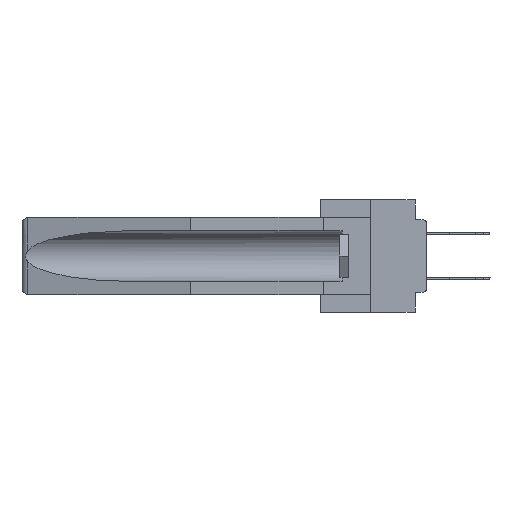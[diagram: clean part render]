
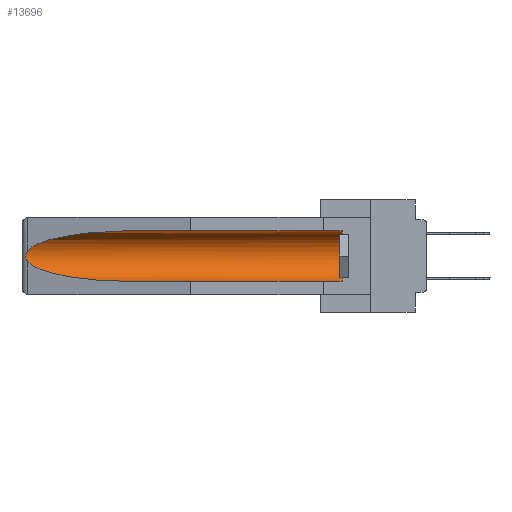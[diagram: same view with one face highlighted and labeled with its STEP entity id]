
A CAD part, left-side view. The second image highlights one B-rep face of the part: STEP entity #13696.
In plain terms, the highlighted cylindrical face has radius 2.857 mm (diameter 5.715 mm), a partial arc.
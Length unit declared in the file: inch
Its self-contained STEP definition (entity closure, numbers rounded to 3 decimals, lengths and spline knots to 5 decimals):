
#3697 = CARTESIAN_POINT ( 'NONE',  ( 0.25451, 1.48313, -0.09465 ) ) ;
#4041 = CARTESIAN_POINT ( 'NONE',  ( 0.26537, 1.52718, -0.14972 ) ) ;
#4140 = CARTESIAN_POINT ( 'NONE',  ( 0.26537, 1.52718, -0.19328 ) ) ;
#4687 = DIRECTION ( 'NONE',  ( 0., 1., 0. ) ) ;
#4761 = EDGE_CURVE ( 'NONE', #7345, #20458, #6407, .T. ) ;
#4946 = B_SPLINE_CURVE_WITH_KNOTS ( 'NONE', 3,
 ( #4041, #6804, #26663, #19474, #11679, #11792, #11461, #6586, #21898, #4140 ),
 .UNSPECIFIED., .F., .F.,
 ( 4, 2, 2, 2, 4 ),
 ( 0., 0.00029, 0.00058, 0.00087, 0.00117 ),
 .UNSPECIFIED. ) ;
#5360 = CARTESIAN_POINT ( 'NONE',  ( 0.155, -0.30754, -0.059 ) ) ;
#5689 = CARTESIAN_POINT ( 'NONE',  ( 0.26537, 1.52718, -0.19328 ) ) ;
#6020 = VERTEX_POINT ( 'NONE', #6176 ) ;
#6176 = CARTESIAN_POINT ( 'NONE',  ( 0.155, 0.126, -0.059 ) ) ;
#6407 = LINE ( 'NONE', #17045, #32652 ) ;
#6586 = CARTESIAN_POINT ( 'NONE',  ( 0.26655, 1.53094, -0.18657 ) ) ;
#6804 = CARTESIAN_POINT ( 'NONE',  ( 0.26597, 1.52961, -0.15275 ) ) ;
#7345 = VERTEX_POINT ( 'NONE', #15353 ) ;
#8483 = ORIENTED_EDGE ( 'NONE', *, *, #4761, .F. ) ;
#9183 = EDGE_CURVE ( 'NONE', #24063, #11106, #10831, .T. ) ;
#9950 = LINE ( 'NONE', #5360, #30214 ) ;
#10102 = EDGE_CURVE ( 'NONE', #7345, #6020, #14023, .T. ) ;
#10831 =( BOUNDED_CURVE ( )  B_SPLINE_CURVE ( 3, ( #16141, #11220, #3697, #11896 ),
 .UNSPECIFIED., .F., .F. ) 
 B_SPLINE_CURVE_WITH_KNOTS ( ( 4, 4 ),
 ( 4.71239, 6.08839 ),
 .UNSPECIFIED. ) 
 CURVE ( )  GEOMETRIC_REPRESENTATION_ITEM ( )  RATIONAL_B_SPLINE_CURVE ( ( 1., 0.848, 0.848, 1. ) ) 
 REPRESENTATION_ITEM ( '' )  );
#11016 = VERTEX_POINT ( 'NONE', #11349 ) ;
#11106 = VERTEX_POINT ( 'NONE', #11783 ) ;
#11220 = CARTESIAN_POINT ( 'NONE',  ( 0.21114, 1.30732, -0.059 ) ) ;
#11349 = CARTESIAN_POINT ( 'NONE',  ( 0.26537, 1.52718, -0.19328 ) ) ;
#11461 = CARTESIAN_POINT ( 'NONE',  ( 0.2673, 1.53269, -0.17917 ) ) ;
#11679 = CARTESIAN_POINT ( 'NONE',  ( 0.2675, 1.53308, -0.16763 ) ) ;
#11783 = CARTESIAN_POINT ( 'NONE',  ( 0.26537, 1.52718, -0.14972 ) ) ;
#11792 = CARTESIAN_POINT ( 'NONE',  ( 0.2675, 1.53308, -0.17534 ) ) ;
#11862 =( BOUNDED_CURVE ( )  B_SPLINE_CURVE ( 3, ( #5689, #23330, #28412, #21090 ),
 .UNSPECIFIED., .F., .F. ) 
 B_SPLINE_CURVE_WITH_KNOTS ( ( 4, 4 ),
 ( 0.1948, 1.5708 ),
 .UNSPECIFIED. ) 
 CURVE ( )  GEOMETRIC_REPRESENTATION_ITEM ( )  RATIONAL_B_SPLINE_CURVE ( ( 1., 0.848, 0.848, 1. ) ) 
 REPRESENTATION_ITEM ( '' )  );
#11896 = CARTESIAN_POINT ( 'NONE',  ( 0.26537, 1.52718, -0.14972 ) ) ;
#12158 = DIRECTION ( 'NONE',  ( 0., 1., 0. ) ) ;
#12189 = CARTESIAN_POINT ( 'NONE',  ( 0.155, 0.126, -0.1715 ) ) ;
#12529 = DIRECTION ( 'NONE',  ( 0., 0., 1. ) ) ;
#12578 = CYLINDRICAL_SURFACE ( 'NONE', #18271, 0.1125 ) ;
#12846 = CARTESIAN_POINT ( 'NONE',  ( 0.155, -0.30754, -0.1715 ) ) ;
#13177 = DIRECTION ( 'NONE',  ( 0., 1., 0. ) ) ;
#13696 = ADVANCED_FACE ( 'NONE', ( #29233 ), #12578, .F. ) ;
#13863 = ORIENTED_EDGE ( 'NONE', *, *, #10102, .T. ) ;
#14023 = CIRCLE ( 'NONE', #27089, 0.1125 ) ;
#15353 = CARTESIAN_POINT ( 'NONE',  ( 0.155, 0.126, -0.284 ) ) ;
#16141 = CARTESIAN_POINT ( 'NONE',  ( 0.155, 1.07973, -0.059 ) ) ;
#17045 = CARTESIAN_POINT ( 'NONE',  ( 0.155, -0.30754, -0.284 ) ) ;
#18271 = AXIS2_PLACEMENT_3D ( 'NONE', #12846, #13177, #18283 ) ;
#18283 = DIRECTION ( 'NONE',  ( 0., 0., 1. ) ) ;
#18339 = CARTESIAN_POINT ( 'NONE',  ( 0.155, 1.07973, -0.059 ) ) ;
#19474 = CARTESIAN_POINT ( 'NONE',  ( 0.2673, 1.5327, -0.16383 ) ) ;
#20458 = VERTEX_POINT ( 'NONE', #25590 ) ;
#21090 = CARTESIAN_POINT ( 'NONE',  ( 0.155, 1.07973, -0.284 ) ) ;
#21898 = CARTESIAN_POINT ( 'NONE',  ( 0.26597, 1.5296, -0.19026 ) ) ;
#23119 = ORIENTED_EDGE ( 'NONE', *, *, #27699, .T. ) ;
#23330 = CARTESIAN_POINT ( 'NONE',  ( 0.25451, 1.48313, -0.24835 ) ) ;
#23549 = ORIENTED_EDGE ( 'NONE', *, *, #31803, .T. ) ;
#24063 = VERTEX_POINT ( 'NONE', #18339 ) ;
#25387 = ORIENTED_EDGE ( 'NONE', *, *, #9183, .T. ) ;
#25590 = CARTESIAN_POINT ( 'NONE',  ( 0.155, 1.07973, -0.284 ) ) ;
#26663 = CARTESIAN_POINT ( 'NONE',  ( 0.26654, 1.53092, -0.15636 ) ) ;
#27089 = AXIS2_PLACEMENT_3D ( 'NONE', #12189, #29931, #12529 ) ;
#27699 = EDGE_CURVE ( 'NONE', #11106, #11016, #4946, .T. ) ;
#28412 = CARTESIAN_POINT ( 'NONE',  ( 0.21114, 1.30732, -0.284 ) ) ;
#29233 = FACE_OUTER_BOUND ( 'NONE', #30801, .T. ) ;
#29931 = DIRECTION ( 'NONE',  ( 0., -1., 0. ) ) ;
#30214 = VECTOR ( 'NONE', #4687, 39.37008 ) ;
#30801 = EDGE_LOOP ( 'NONE', ( #25387, #23119, #23549, #8483, #13863, #32534 ) ) ;
#31658 = EDGE_CURVE ( 'NONE', #6020, #24063, #9950, .T. ) ;
#31803 = EDGE_CURVE ( 'NONE', #11016, #20458, #11862, .T. ) ;
#32534 = ORIENTED_EDGE ( 'NONE', *, *, #31658, .T. ) ;
#32652 = VECTOR ( 'NONE', #12158, 39.37008 ) ;
